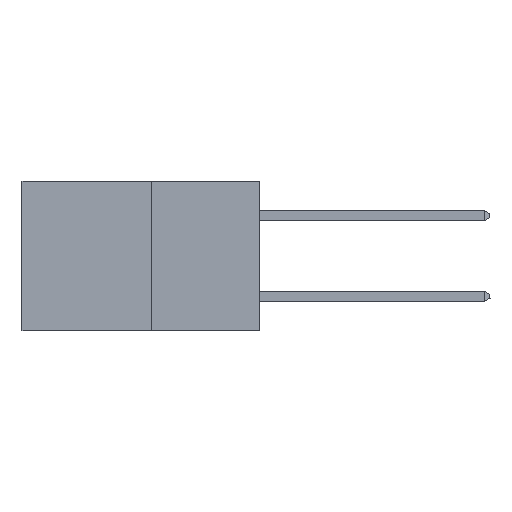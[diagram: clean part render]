
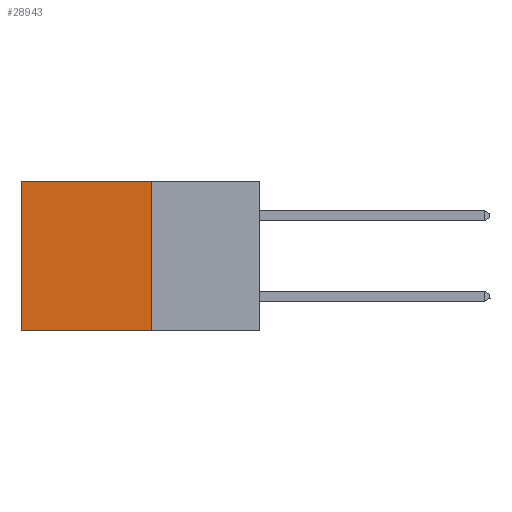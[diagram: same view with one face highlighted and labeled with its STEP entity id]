
A CAD part, left-side view. The second image highlights one B-rep face of the part: STEP entity #28943.
In plain terms, the highlighted planar face has unit normal (-1, 0, 0).
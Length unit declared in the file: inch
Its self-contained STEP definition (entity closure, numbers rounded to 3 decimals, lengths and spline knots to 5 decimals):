
#340 = AXIS2_PLACEMENT_3D ( 'NONE', #27333, #4292, #20629 ) ;
#369 = ORIENTED_EDGE ( 'NONE', *, *, #18706, .F. ) ;
#1122 = VECTOR ( 'NONE', #26031, 39.37008 ) ;
#1812 = EDGE_CURVE ( 'NONE', #22655, #8735, #15155, .T. ) ;
#2264 = CARTESIAN_POINT ( 'NONE',  ( 0.277, 0.27, -0.37 ) ) ;
#2480 = FACE_OUTER_BOUND ( 'NONE', #24578, .T. ) ;
#2774 = EDGE_CURVE ( 'NONE', #22655, #14112, #13644, .T. ) ;
#4191 = PLANE ( 'NONE',  #340 ) ;
#4292 = DIRECTION ( 'NONE',  ( 1., 0., 0. ) ) ;
#4439 = VERTEX_POINT ( 'NONE', #23062 ) ;
#4661 = DIRECTION ( 'NONE',  ( 0., 1., 0. ) ) ;
#6947 = CARTESIAN_POINT ( 'NONE',  ( 0.277, 0.27, 0. ) ) ;
#8735 = VERTEX_POINT ( 'NONE', #26251 ) ;
#8830 = LINE ( 'NONE', #16710, #27840 ) ;
#9875 = DIRECTION ( 'NONE',  ( 0., 0., -1. ) ) ;
#11356 = EDGE_CURVE ( 'NONE', #8735, #4439, #8830, .T. ) ;
#12351 = CARTESIAN_POINT ( 'NONE',  ( 0.277, 0.27, 0. ) ) ;
#13644 = LINE ( 'NONE', #26192, #1122 ) ;
#14112 = VERTEX_POINT ( 'NONE', #17320 ) ;
#15155 = LINE ( 'NONE', #6947, #26636 ) ;
#16293 = DIRECTION ( 'NONE',  ( 0., 1., 0. ) ) ;
#16710 = CARTESIAN_POINT ( 'NONE',  ( 0.277, 0.59, -0.37 ) ) ;
#17320 = CARTESIAN_POINT ( 'NONE',  ( 0.277, 0.27, -0.37 ) ) ;
#17410 = VECTOR ( 'NONE', #4661, 39.37008 ) ;
#18706 = EDGE_CURVE ( 'NONE', #14112, #4439, #29478, .T. ) ;
#20629 = DIRECTION ( 'NONE',  ( 0., 0., -1. ) ) ;
#22655 = VERTEX_POINT ( 'NONE', #12351 ) ;
#23062 = CARTESIAN_POINT ( 'NONE',  ( 0.277, 0.59, -0.37 ) ) ;
#24578 = EDGE_LOOP ( 'NONE', ( #25097, #369, #27261, #27733 ) ) ;
#25097 = ORIENTED_EDGE ( 'NONE', *, *, #11356, .T. ) ;
#26031 = DIRECTION ( 'NONE',  ( 0., 0., -1. ) ) ;
#26192 = CARTESIAN_POINT ( 'NONE',  ( 0.277, 0.27, -0.37 ) ) ;
#26251 = CARTESIAN_POINT ( 'NONE',  ( 0.277, 0.59, 0. ) ) ;
#26636 = VECTOR ( 'NONE', #16293, 39.37008 ) ;
#27261 = ORIENTED_EDGE ( 'NONE', *, *, #2774, .F. ) ;
#27333 = CARTESIAN_POINT ( 'NONE',  ( 0.277, 0.27, -0.37 ) ) ;
#27733 = ORIENTED_EDGE ( 'NONE', *, *, #1812, .T. ) ;
#27840 = VECTOR ( 'NONE', #9875, 39.37008 ) ;
#28943 = ADVANCED_FACE ( 'NONE', ( #2480 ), #4191, .F. ) ;
#29478 = LINE ( 'NONE', #2264, #17410 ) ;
